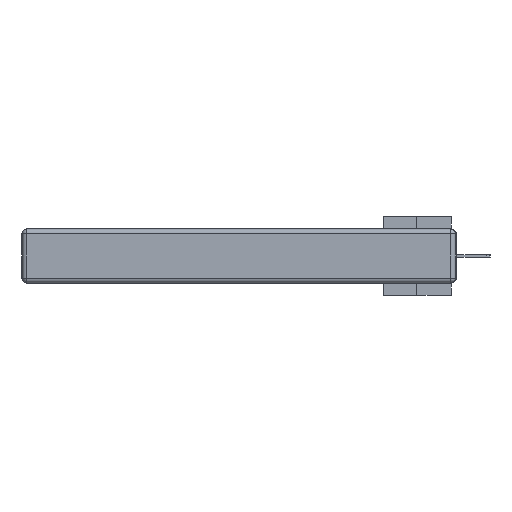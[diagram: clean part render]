
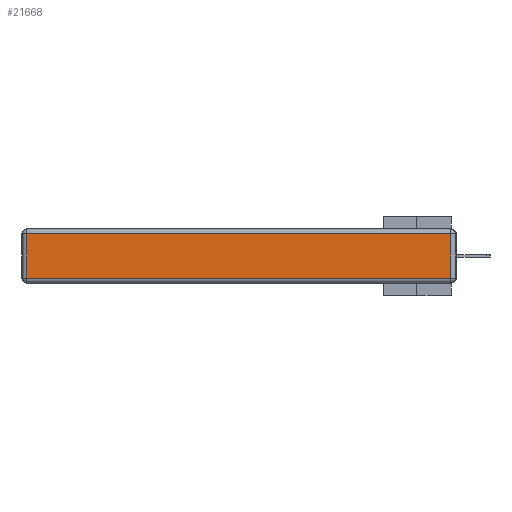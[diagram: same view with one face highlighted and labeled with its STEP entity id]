
A CAD part, left-side view. The second image highlights one B-rep face of the part: STEP entity #21668.
In plain terms, the highlighted planar face has unit normal (-1, 0, 0).
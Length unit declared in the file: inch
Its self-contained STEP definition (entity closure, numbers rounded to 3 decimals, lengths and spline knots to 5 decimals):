
#4107 = ORIENTED_EDGE ( 'NONE', *, *, #18646, .T. ) ;
#5294 = CARTESIAN_POINT ( 'NONE',  ( 0., 0.03, -0.343 ) ) ;
#5862 = DIRECTION ( 'NONE',  ( 0., 0., 1. ) ) ;
#5876 = CARTESIAN_POINT ( 'NONE',  ( 0., 0., -0.343 ) ) ;
#6493 = EDGE_CURVE ( 'NONE', #22004, #8583, #15388, .T. ) ;
#6973 = AXIS2_PLACEMENT_3D ( 'NONE', #5876, #29070, #32122 ) ;
#7102 = EDGE_CURVE ( 'NONE', #32166, #22004, #20607, .T. ) ;
#8583 = VERTEX_POINT ( 'NONE', #29487 ) ;
#8960 = FACE_OUTER_BOUND ( 'NONE', #23787, .T. ) ;
#9130 = DIRECTION ( 'NONE',  ( 0., -1., 0. ) ) ;
#10959 = VECTOR ( 'NONE', #35666, 39.37008 ) ;
#14821 = CARTESIAN_POINT ( 'NONE',  ( 0., 2.75, -0.03 ) ) ;
#15151 = CARTESIAN_POINT ( 'NONE',  ( 0., 2.72, -0.343 ) ) ;
#15388 = LINE ( 'NONE', #14821, #10959 ) ;
#16506 = ORIENTED_EDGE ( 'NONE', *, *, #7102, .T. ) ;
#16910 = ORIENTED_EDGE ( 'NONE', *, *, #25104, .T. ) ;
#17477 = CARTESIAN_POINT ( 'NONE',  ( 0., 0.03, -0.03 ) ) ;
#18646 = EDGE_CURVE ( 'NONE', #18906, #32166, #20615, .T. ) ;
#18906 = VERTEX_POINT ( 'NONE', #19816 ) ;
#19816 = CARTESIAN_POINT ( 'NONE',  ( 0., 2.72, -0.313 ) ) ;
#20607 = LINE ( 'NONE', #5294, #33614 ) ;
#20615 = LINE ( 'NONE', #32497, #32568 ) ;
#21668 = ADVANCED_FACE ( 'NONE', ( #8960 ), #37854, .T. ) ;
#22004 = VERTEX_POINT ( 'NONE', #17477 ) ;
#22178 = CARTESIAN_POINT ( 'NONE',  ( 0., 0.03, -0.313 ) ) ;
#23787 = EDGE_LOOP ( 'NONE', ( #4107, #16506, #33629, #16910 ) ) ;
#25104 = EDGE_CURVE ( 'NONE', #8583, #18906, #29528, .T. ) ;
#26844 = DIRECTION ( 'NONE',  ( 0., 0., -1. ) ) ;
#29070 = DIRECTION ( 'NONE',  ( -1., 0., 0. ) ) ;
#29487 = CARTESIAN_POINT ( 'NONE',  ( 0., 2.72, -0.03 ) ) ;
#29528 = LINE ( 'NONE', #15151, #34006 ) ;
#32122 = DIRECTION ( 'NONE',  ( 0., 0., 1. ) ) ;
#32166 = VERTEX_POINT ( 'NONE', #22178 ) ;
#32497 = CARTESIAN_POINT ( 'NONE',  ( 0., 0., -0.313 ) ) ;
#32568 = VECTOR ( 'NONE', #9130, 39.37008 ) ;
#33614 = VECTOR ( 'NONE', #5862, 39.37008 ) ;
#33629 = ORIENTED_EDGE ( 'NONE', *, *, #6493, .T. ) ;
#34006 = VECTOR ( 'NONE', #26844, 39.37008 ) ;
#35666 = DIRECTION ( 'NONE',  ( 0., 1., 0. ) ) ;
#37854 = PLANE ( 'NONE',  #6973 ) ;
